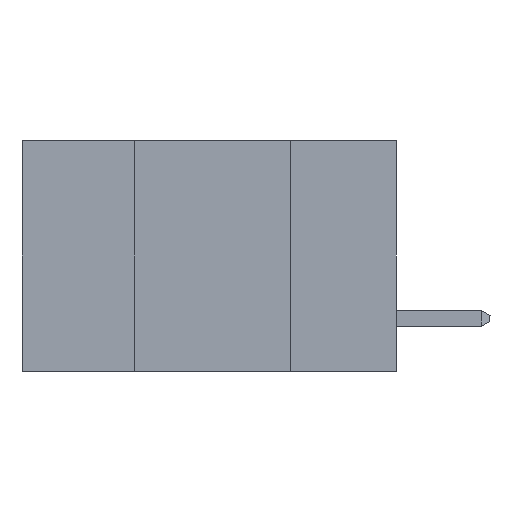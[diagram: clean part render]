
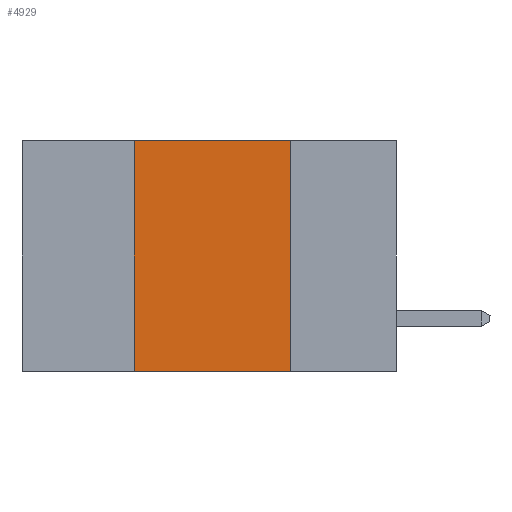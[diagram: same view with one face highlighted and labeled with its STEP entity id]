
A CAD part, left-side view. The second image highlights one B-rep face of the part: STEP entity #4929.
In plain terms, the highlighted planar face has unit normal (-1, 0, 0).
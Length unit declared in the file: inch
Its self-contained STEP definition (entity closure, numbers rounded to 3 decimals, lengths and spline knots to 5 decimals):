
#277 = CARTESIAN_POINT ( 'NONE',  ( 0., 0.17, -0.37 ) ) ;
#1016 = CARTESIAN_POINT ( 'NONE',  ( 0., 0.6, -0.37 ) ) ;
#1964 = EDGE_CURVE ( 'NONE', #10239, #3556, #9706, .T. ) ;
#2153 = DIRECTION ( 'NONE',  ( 1., 0., 0. ) ) ;
#2261 = CARTESIAN_POINT ( 'NONE',  ( 0., 0.17, -0.37 ) ) ;
#2308 = LINE ( 'NONE', #6302, #6513 ) ;
#3032 = ORIENTED_EDGE ( 'NONE', *, *, #4583, .T. ) ;
#3208 = DIRECTION ( 'NONE',  ( 0., 0., 1. ) ) ;
#3376 = AXIS2_PLACEMENT_3D ( 'NONE', #9103, #2153, #11836 ) ;
#3407 = EDGE_CURVE ( 'NONE', #3556, #7894, #3514, .T. ) ;
#3514 = LINE ( 'NONE', #277, #3986 ) ;
#3556 = VERTEX_POINT ( 'NONE', #8591 ) ;
#3726 = DIRECTION ( 'NONE',  ( 0., -1., 0. ) ) ;
#3809 = LINE ( 'NONE', #1016, #12712 ) ;
#3888 = VERTEX_POINT ( 'NONE', #11553 ) ;
#3986 = VECTOR ( 'NONE', #12285, 39.37008 ) ;
#4583 = EDGE_CURVE ( 'NONE', #3888, #7894, #3809, .T. ) ;
#4929 = ADVANCED_FACE ( 'NONE', ( #4964 ), #8920, .F. ) ;
#4964 = FACE_OUTER_BOUND ( 'NONE', #5726, .T. ) ;
#5051 = DIRECTION ( 'NONE',  ( 0., -1., 0. ) ) ;
#5253 = ORIENTED_EDGE ( 'NONE', *, *, #9616, .F. ) ;
#5726 = EDGE_LOOP ( 'NONE', ( #8583, #6005, #5253, #3032 ) ) ;
#6005 = ORIENTED_EDGE ( 'NONE', *, *, #1964, .F. ) ;
#6233 = VECTOR ( 'NONE', #3726, 39.37008 ) ;
#6302 = CARTESIAN_POINT ( 'NONE',  ( 0., 0.42, -0.37 ) ) ;
#6513 = VECTOR ( 'NONE', #3208, 39.37008 ) ;
#7894 = VERTEX_POINT ( 'NONE', #2261 ) ;
#8583 = ORIENTED_EDGE ( 'NONE', *, *, #3407, .F. ) ;
#8591 = CARTESIAN_POINT ( 'NONE',  ( 0., 0.17, 0. ) ) ;
#8920 = PLANE ( 'NONE',  #3376 ) ;
#9103 = CARTESIAN_POINT ( 'NONE',  ( 0., 0.6, 0. ) ) ;
#9448 = CARTESIAN_POINT ( 'NONE',  ( 0., 0.6, 0. ) ) ;
#9616 = EDGE_CURVE ( 'NONE', #3888, #10239, #2308, .T. ) ;
#9706 = LINE ( 'NONE', #9448, #6233 ) ;
#10239 = VERTEX_POINT ( 'NONE', #10670 ) ;
#10670 = CARTESIAN_POINT ( 'NONE',  ( 0., 0.42, 0. ) ) ;
#11553 = CARTESIAN_POINT ( 'NONE',  ( 0., 0.42, -0.37 ) ) ;
#11836 = DIRECTION ( 'NONE',  ( 0., 0., -1. ) ) ;
#12285 = DIRECTION ( 'NONE',  ( 0., 0., -1. ) ) ;
#12712 = VECTOR ( 'NONE', #5051, 39.37008 ) ;
